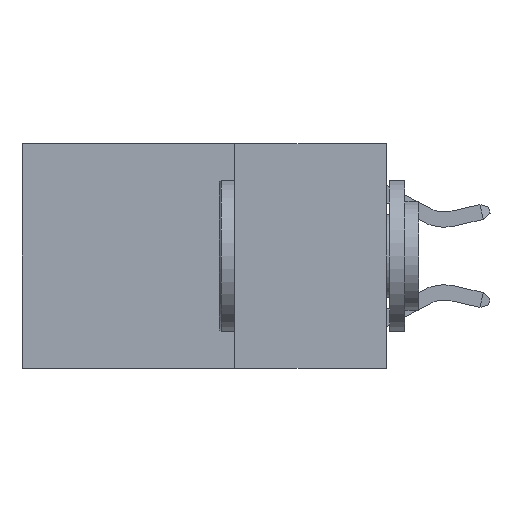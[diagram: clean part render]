
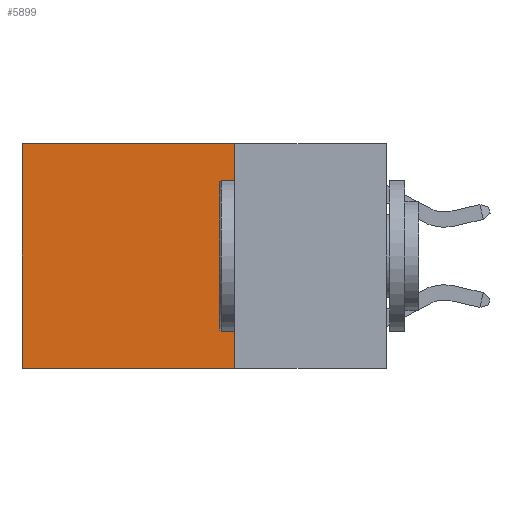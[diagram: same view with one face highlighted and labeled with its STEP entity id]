
A CAD part, left-side view. The second image highlights one B-rep face of the part: STEP entity #5899.
In plain terms, the highlighted planar face has unit normal (-1, 0, 0).
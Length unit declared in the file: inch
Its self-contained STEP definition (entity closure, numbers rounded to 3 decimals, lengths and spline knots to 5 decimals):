
#231 = EDGE_CURVE ( 'NONE', #13756, #4419, #4030, .T. ) ;
#252 = ORIENTED_EDGE ( 'NONE', *, *, #12852, .F. ) ;
#359 = CARTESIAN_POINT ( 'NONE',  ( 0.2625, 0.25, -0.37 ) ) ;
#716 = VECTOR ( 'NONE', #20364, 39.37008 ) ;
#1197 = VERTEX_POINT ( 'NONE', #6314 ) ;
#1482 = DIRECTION ( 'NONE',  ( 0., 0., -1. ) ) ;
#4030 = LINE ( 'NONE', #6237, #5021 ) ;
#4419 = VERTEX_POINT ( 'NONE', #8477 ) ;
#5021 = VECTOR ( 'NONE', #16022, 39.37008 ) ;
#5543 = LINE ( 'NONE', #7319, #716 ) ;
#5700 = CARTESIAN_POINT ( 'NONE',  ( 0.2625, 0.25, 0. ) ) ;
#5899 = ADVANCED_FACE ( 'NONE', ( #13872 ), #14992, .F. ) ;
#5947 = VERTEX_POINT ( 'NONE', #5700 ) ;
#6237 = CARTESIAN_POINT ( 'NONE',  ( 0.2625, 0.25, -0.37 ) ) ;
#6314 = CARTESIAN_POINT ( 'NONE',  ( 0.2625, 0.6, 0. ) ) ;
#6324 = VECTOR ( 'NONE', #1482, 39.37008 ) ;
#6779 = DIRECTION ( 'NONE',  ( 1., 0., 0. ) ) ;
#7093 = ORIENTED_EDGE ( 'NONE', *, *, #17778, .T. ) ;
#7319 = CARTESIAN_POINT ( 'NONE',  ( 0.2625, 0.25, 0. ) ) ;
#7322 = ORIENTED_EDGE ( 'NONE', *, *, #231, .F. ) ;
#7814 = EDGE_LOOP ( 'NONE', ( #13317, #7322, #252, #7093 ) ) ;
#8006 = CARTESIAN_POINT ( 'NONE',  ( 0.2625, 0.25, 0. ) ) ;
#8429 = AXIS2_PLACEMENT_3D ( 'NONE', #10126, #6779, #11686 ) ;
#8477 = CARTESIAN_POINT ( 'NONE',  ( 0.2625, 0.6, -0.37 ) ) ;
#8878 = LINE ( 'NONE', #8006, #6324 ) ;
#9204 = DIRECTION ( 'NONE',  ( 0., 0., -1. ) ) ;
#10126 = CARTESIAN_POINT ( 'NONE',  ( 0.2625, 0.25, 0. ) ) ;
#11686 = DIRECTION ( 'NONE',  ( 0., 0., -1. ) ) ;
#12852 = EDGE_CURVE ( 'NONE', #5947, #13756, #8878, .T. ) ;
#13317 = ORIENTED_EDGE ( 'NONE', *, *, #13443, .T. ) ;
#13443 = EDGE_CURVE ( 'NONE', #1197, #4419, #16202, .T. ) ;
#13756 = VERTEX_POINT ( 'NONE', #359 ) ;
#13872 = FACE_OUTER_BOUND ( 'NONE', #7814, .T. ) ;
#14992 = PLANE ( 'NONE',  #8429 ) ;
#16022 = DIRECTION ( 'NONE',  ( 0., 1., 0. ) ) ;
#16202 = LINE ( 'NONE', #17547, #19490 ) ;
#17547 = CARTESIAN_POINT ( 'NONE',  ( 0.2625, 0.6, 0. ) ) ;
#17778 = EDGE_CURVE ( 'NONE', #5947, #1197, #5543, .T. ) ;
#19490 = VECTOR ( 'NONE', #9204, 39.37008 ) ;
#20364 = DIRECTION ( 'NONE',  ( 0., 1., 0. ) ) ;
